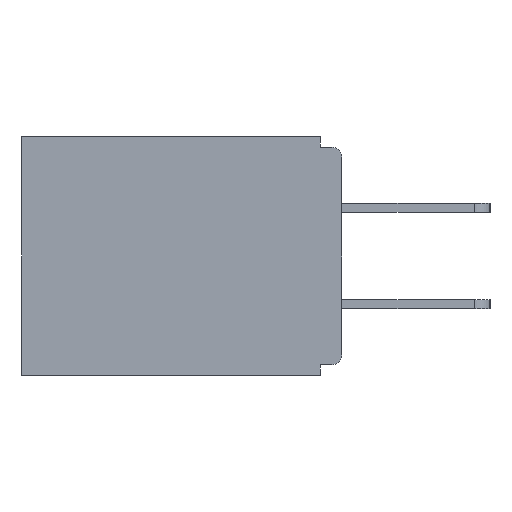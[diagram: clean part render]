
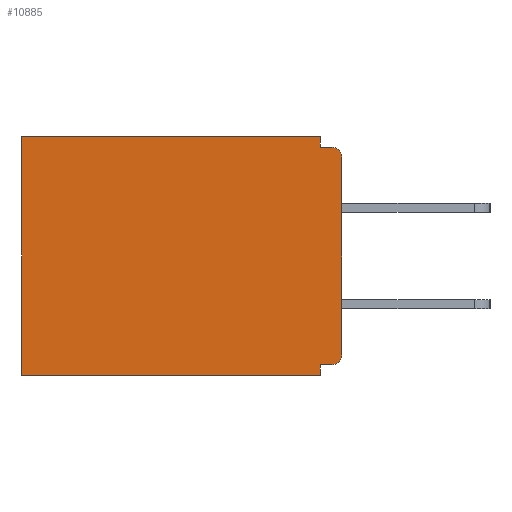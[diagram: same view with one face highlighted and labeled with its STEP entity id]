
A CAD part, left-side view. The second image highlights one B-rep face of the part: STEP entity #10885.
In plain terms, the highlighted planar face has unit normal (-1, 0, 0).
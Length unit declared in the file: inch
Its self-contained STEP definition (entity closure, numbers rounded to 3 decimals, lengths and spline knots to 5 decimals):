
#60 = VECTOR ( 'NONE', #3704, 39.37008 ) ;
#178 = LINE ( 'NONE', #8947, #11603 ) ;
#230 = DIRECTION ( 'NONE',  ( 0., 0., -1. ) ) ;
#552 = VERTEX_POINT ( 'NONE', #9447 ) ;
#710 = CARTESIAN_POINT ( 'NONE',  ( 0.298, 0.031, -0.343 ) ) ;
#895 = CIRCLE ( 'NONE', #14259, 0.015 ) ;
#961 = DIRECTION ( 'NONE',  ( 0., 1., 0. ) ) ;
#1391 = ORIENTED_EDGE ( 'NONE', *, *, #6920, .F. ) ;
#1444 = PLANE ( 'NONE',  #2570 ) ;
#1521 = EDGE_CURVE ( 'NONE', #552, #7770, #7679, .T. ) ;
#2132 = DIRECTION ( 'NONE',  ( -1., 0., 0. ) ) ;
#2290 = EDGE_CURVE ( 'NONE', #5477, #8182, #895, .T. ) ;
#2426 = LINE ( 'NONE', #3380, #11605 ) ;
#2570 = AXIS2_PLACEMENT_3D ( 'NONE', #3724, #6956, #4743 ) ;
#2578 = CARTESIAN_POINT ( 'NONE',  ( 0.298, 0., 0. ) ) ;
#2781 = CARTESIAN_POINT ( 'NONE',  ( 0.298, 0.46, 0. ) ) ;
#2835 = ORIENTED_EDGE ( 'NONE', *, *, #4264, .F. ) ;
#2885 = DIRECTION ( 'NONE',  ( 0., -1., 0. ) ) ;
#3157 = CARTESIAN_POINT ( 'NONE',  ( 0.298, 0.031, -0.015 ) ) ;
#3265 = LINE ( 'NONE', #5125, #13804 ) ;
#3327 = ORIENTED_EDGE ( 'NONE', *, *, #13115, .F. ) ;
#3380 = CARTESIAN_POINT ( 'NONE',  ( 0.298, 0., -0.343 ) ) ;
#3387 = ORIENTED_EDGE ( 'NONE', *, *, #2290, .T. ) ;
#3482 = DIRECTION ( 'NONE',  ( 0., 1., 0. ) ) ;
#3704 = DIRECTION ( 'NONE',  ( 0., 1., 0. ) ) ;
#3724 = CARTESIAN_POINT ( 'NONE',  ( 0.298, 0., 0. ) ) ;
#3781 = EDGE_CURVE ( 'NONE', #7770, #4556, #178, .T. ) ;
#3878 = VERTEX_POINT ( 'NONE', #13525 ) ;
#3982 = ORIENTED_EDGE ( 'NONE', *, *, #8741, .T. ) ;
#4082 = ORIENTED_EDGE ( 'NONE', *, *, #8511, .F. ) ;
#4264 = EDGE_CURVE ( 'NONE', #7694, #4556, #2426, .T. ) ;
#4445 = VECTOR ( 'NONE', #5443, 39.37008 ) ;
#4534 = EDGE_CURVE ( 'NONE', #5477, #11300, #12619, .T. ) ;
#4556 = VERTEX_POINT ( 'NONE', #9976 ) ;
#4681 = ORIENTED_EDGE ( 'NONE', *, *, #7515, .F. ) ;
#4743 = DIRECTION ( 'NONE',  ( 0., 0., -1. ) ) ;
#4872 = CARTESIAN_POINT ( 'NONE',  ( 0.298, 0., -0.03 ) ) ;
#5012 = LINE ( 'NONE', #12853, #11932 ) ;
#5111 = CIRCLE ( 'NONE', #13662, 0.015 ) ;
#5125 = CARTESIAN_POINT ( 'NONE',  ( 0.298, 0.031, -0.343 ) ) ;
#5443 = DIRECTION ( 'NONE',  ( 0., 0., -1. ) ) ;
#5477 = VERTEX_POINT ( 'NONE', #13869 ) ;
#6432 = CARTESIAN_POINT ( 'NONE',  ( 0.298, 0., -0.328 ) ) ;
#6614 = CARTESIAN_POINT ( 'NONE',  ( 0.298, 0.015, -0.03 ) ) ;
#6866 = CARTESIAN_POINT ( 'NONE',  ( 0.298, 0., 0. ) ) ;
#6920 = EDGE_CURVE ( 'NONE', #7776, #8182, #12258, .T. ) ;
#6956 = DIRECTION ( 'NONE',  ( 1., 0., 0. ) ) ;
#7515 = EDGE_CURVE ( 'NONE', #11300, #7694, #3265, .T. ) ;
#7554 = ORIENTED_EDGE ( 'NONE', *, *, #1521, .T. ) ;
#7679 = LINE ( 'NONE', #2578, #60 ) ;
#7694 = VERTEX_POINT ( 'NONE', #9861 ) ;
#7757 = CARTESIAN_POINT ( 'NONE',  ( 0.298, 0., -0.313 ) ) ;
#7770 = VERTEX_POINT ( 'NONE', #2781 ) ;
#7776 = VERTEX_POINT ( 'NONE', #4872 ) ;
#8169 = FACE_OUTER_BOUND ( 'NONE', #13762, .T. ) ;
#8182 = VERTEX_POINT ( 'NONE', #7757 ) ;
#8511 = EDGE_CURVE ( 'NONE', #552, #11578, #10640, .T. ) ;
#8687 = ORIENTED_EDGE ( 'NONE', *, *, #4534, .F. ) ;
#8741 = EDGE_CURVE ( 'NONE', #7776, #3878, #5111, .T. ) ;
#8947 = CARTESIAN_POINT ( 'NONE',  ( 0.298, 0.46, 0. ) ) ;
#9447 = CARTESIAN_POINT ( 'NONE',  ( 0.298, 0.031, 0. ) ) ;
#9472 = DIRECTION ( 'NONE',  ( 0., 0., -1. ) ) ;
#9861 = CARTESIAN_POINT ( 'NONE',  ( 0.298, 0.031, -0.343 ) ) ;
#9976 = CARTESIAN_POINT ( 'NONE',  ( 0.298, 0.46, -0.343 ) ) ;
#10002 = DIRECTION ( 'NONE',  ( 0., 0., -1. ) ) ;
#10177 = VECTOR ( 'NONE', #230, 39.37008 ) ;
#10640 = LINE ( 'NONE', #710, #4445 ) ;
#10662 = DIRECTION ( 'NONE',  ( 0., 0., -1. ) ) ;
#10885 = ADVANCED_FACE ( 'NONE', ( #8169 ), #1444, .F. ) ;
#11106 = ORIENTED_EDGE ( 'NONE', *, *, #3781, .T. ) ;
#11252 = VECTOR ( 'NONE', #961, 39.37008 ) ;
#11300 = VERTEX_POINT ( 'NONE', #13517 ) ;
#11578 = VERTEX_POINT ( 'NONE', #3157 ) ;
#11603 = VECTOR ( 'NONE', #10002, 39.37008 ) ;
#11605 = VECTOR ( 'NONE', #3482, 39.37008 ) ;
#11932 = VECTOR ( 'NONE', #2885, 39.37008 ) ;
#12258 = LINE ( 'NONE', #6866, #10177 ) ;
#12619 = LINE ( 'NONE', #6432, #11252 ) ;
#12711 = DIRECTION ( 'NONE',  ( -1., 0., 0. ) ) ;
#12853 = CARTESIAN_POINT ( 'NONE',  ( 0.298, 0., -0.015 ) ) ;
#13115 = EDGE_CURVE ( 'NONE', #11578, #3878, #5012, .T. ) ;
#13280 = DIRECTION ( 'NONE',  ( 0., 0., -1. ) ) ;
#13517 = CARTESIAN_POINT ( 'NONE',  ( 0.298, 0.031, -0.328 ) ) ;
#13525 = CARTESIAN_POINT ( 'NONE',  ( 0.298, 0.015, -0.015 ) ) ;
#13662 = AXIS2_PLACEMENT_3D ( 'NONE', #6614, #2132, #13280 ) ;
#13762 = EDGE_LOOP ( 'NONE', ( #3982, #3327, #4082, #7554, #11106, #2835, #4681, #8687, #3387, #1391 ) ) ;
#13804 = VECTOR ( 'NONE', #9472, 39.37008 ) ;
#13869 = CARTESIAN_POINT ( 'NONE',  ( 0.298, 0.015, -0.328 ) ) ;
#13948 = CARTESIAN_POINT ( 'NONE',  ( 0.298, 0.015, -0.313 ) ) ;
#14259 = AXIS2_PLACEMENT_3D ( 'NONE', #13948, #12711, #10662 ) ;
